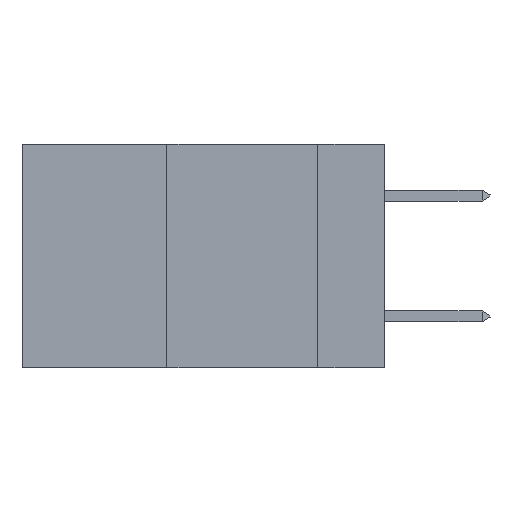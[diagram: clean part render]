
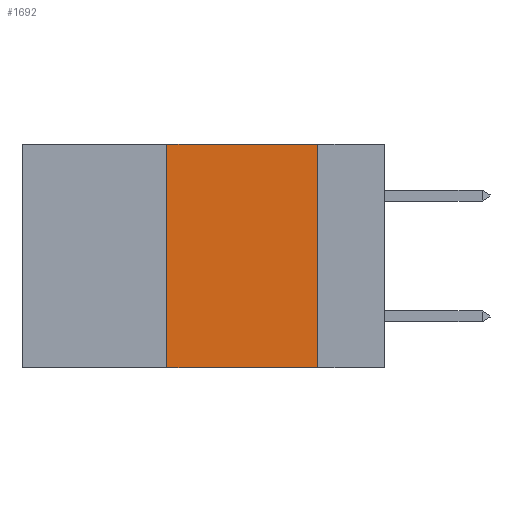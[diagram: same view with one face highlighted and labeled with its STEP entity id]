
A CAD part, left-side view. The second image highlights one B-rep face of the part: STEP entity #1692.
In plain terms, the highlighted planar face has unit normal (-1, 0, 0).
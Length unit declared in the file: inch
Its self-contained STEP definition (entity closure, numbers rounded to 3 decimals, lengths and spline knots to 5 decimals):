
#28 = EDGE_LOOP ( 'NONE', ( #16075, #17725, #22322, #9494 ) ) ;
#1247 = PLANE ( 'NONE',  #8957 ) ;
#1692 = ADVANCED_FACE ( 'NONE', ( #3674 ), #1247, .F. ) ;
#2497 = CARTESIAN_POINT ( 'NONE',  ( 0., 0.36, -0.37 ) ) ;
#3205 = EDGE_CURVE ( 'NONE', #10426, #15615, #12684, .T. ) ;
#3674 = FACE_OUTER_BOUND ( 'NONE', #28, .T. ) ;
#4587 = VERTEX_POINT ( 'NONE', #5890 ) ;
#5890 = CARTESIAN_POINT ( 'NONE',  ( 0., 0.11, 0. ) ) ;
#6077 = VERTEX_POINT ( 'NONE', #6507 ) ;
#6507 = CARTESIAN_POINT ( 'NONE',  ( 0., 0.36, 0. ) ) ;
#6809 = CARTESIAN_POINT ( 'NONE',  ( 0., 0.11, 0. ) ) ;
#8557 = LINE ( 'NONE', #6809, #21389 ) ;
#8581 = VECTOR ( 'NONE', #9090, 39.37008 ) ;
#8957 = AXIS2_PLACEMENT_3D ( 'NONE', #20529, #22252, #11811 ) ;
#9090 = DIRECTION ( 'NONE',  ( 0., -1., 0. ) ) ;
#9174 = CARTESIAN_POINT ( 'NONE',  ( 0., 0.36, 0. ) ) ;
#9494 = ORIENTED_EDGE ( 'NONE', *, *, #3205, .T. ) ;
#9577 = EDGE_CURVE ( 'NONE', #6077, #4587, #16390, .T. ) ;
#10426 = VERTEX_POINT ( 'NONE', #2497 ) ;
#10456 = CARTESIAN_POINT ( 'NONE',  ( 0., 0.11, -0.37 ) ) ;
#10507 = CARTESIAN_POINT ( 'NONE',  ( 0., 0.6, 0. ) ) ;
#10558 = LINE ( 'NONE', #9174, #19308 ) ;
#11811 = DIRECTION ( 'NONE',  ( 0., 0., -1. ) ) ;
#12684 = LINE ( 'NONE', #19594, #8581 ) ;
#12701 = DIRECTION ( 'NONE',  ( 0., 0., 1. ) ) ;
#15564 = DIRECTION ( 'NONE',  ( 0., 0., -1. ) ) ;
#15615 = VERTEX_POINT ( 'NONE', #10456 ) ;
#16075 = ORIENTED_EDGE ( 'NONE', *, *, #21957, .F. ) ;
#16390 = LINE ( 'NONE', #10507, #21011 ) ;
#17545 = DIRECTION ( 'NONE',  ( 0., -1., 0. ) ) ;
#17725 = ORIENTED_EDGE ( 'NONE', *, *, #9577, .F. ) ;
#19308 = VECTOR ( 'NONE', #12701, 39.37008 ) ;
#19594 = CARTESIAN_POINT ( 'NONE',  ( 0., 0.6, -0.37 ) ) ;
#19663 = EDGE_CURVE ( 'NONE', #10426, #6077, #10558, .T. ) ;
#20529 = CARTESIAN_POINT ( 'NONE',  ( 0., 0.6, 0. ) ) ;
#21011 = VECTOR ( 'NONE', #17545, 39.37008 ) ;
#21389 = VECTOR ( 'NONE', #15564, 39.37008 ) ;
#21957 = EDGE_CURVE ( 'NONE', #4587, #15615, #8557, .T. ) ;
#22252 = DIRECTION ( 'NONE',  ( 1., 0., 0. ) ) ;
#22322 = ORIENTED_EDGE ( 'NONE', *, *, #19663, .F. ) ;
